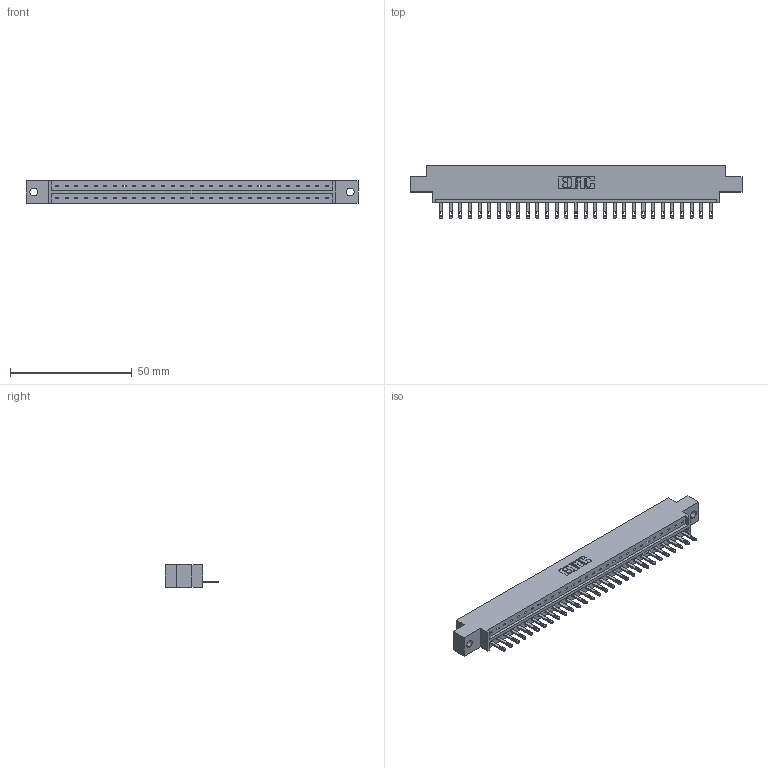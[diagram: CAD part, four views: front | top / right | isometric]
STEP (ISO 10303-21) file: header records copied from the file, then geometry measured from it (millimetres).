
FILE_DESCRIPTION (( 'STEP AP203' ), '1' );
FILE_NAME ('833-029-500-602.STEP', '2020-06-02T10:21:47', ( '' ), ( '' ), 'SwSTEP 2.0', 'SolidWorks 2020', '' );
FILE_SCHEMA (( 'CONFIG_CONTROL_DESIGN' ));
Length unit declared in the file: inch
Products named in the file (3): 345-292-001_345-293-100; 833 Part_Offset - .128 Dia; 833-029-500-602
Assembly tree (30 placements, depth 2):
  833-029-500-602
    833 Part_Offset - .128 Dia
    345-292-001_345-293-100  x29
Bounding box: 136.45 x 21.85 x 9.4 mm (x, y, z)
Volume: 13372.3 mm3; surface area: 14379.7 mm2
Topology: 30 solids, 30 shells, 1684 faces, 5195 edges, 3462 vertices
Faces by surface type: plane 1118, cylinder 566
Entity records: 19475 total; most frequent: CARTESIAN_POINT 3369, ORIENTED_EDGE 3334, DIRECTION 2869, EDGE_CURVE 1667, LINE 1535, VECTOR 1535, VERTEX_POINT 1110, AXIS2_PLACEMENT_3D 667
